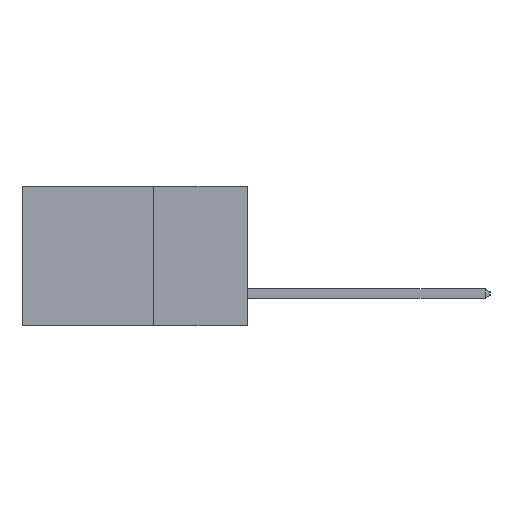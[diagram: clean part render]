
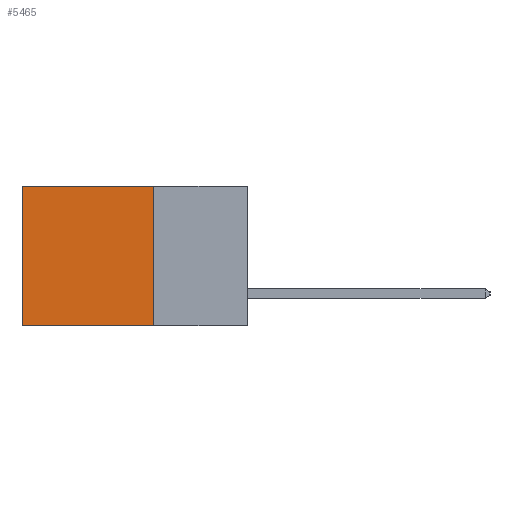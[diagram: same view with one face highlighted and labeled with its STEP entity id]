
A CAD part, left-side view. The second image highlights one B-rep face of the part: STEP entity #5465.
In plain terms, the highlighted planar face has unit normal (-1, 0, 0).
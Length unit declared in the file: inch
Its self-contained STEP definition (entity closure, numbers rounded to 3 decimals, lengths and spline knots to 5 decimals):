
#389 = ORIENTED_EDGE ( 'NONE', *, *, #894, .F. ) ;
#746 = LINE ( 'NONE', #4084, #8252 ) ;
#894 = EDGE_CURVE ( 'NONE', #5451, #9599, #11026, .T. ) ;
#908 = ORIENTED_EDGE ( 'NONE', *, *, #3267, .F. ) ;
#2327 = DIRECTION ( 'NONE',  ( 0., 0., -1. ) ) ;
#2341 = DIRECTION ( 'NONE',  ( 1., 0., 0. ) ) ;
#2351 = CARTESIAN_POINT ( 'NONE',  ( 0.2615, 0.25, -0.37 ) ) ;
#2366 = PLANE ( 'NONE',  #8957 ) ;
#2513 = CARTESIAN_POINT ( 'NONE',  ( 0.2615, 0.6, -0.37 ) ) ;
#2515 = ORIENTED_EDGE ( 'NONE', *, *, #6167, .T. ) ;
#2605 = CARTESIAN_POINT ( 'NONE',  ( 0.2615, 0.25, 0. ) ) ;
#3267 = EDGE_CURVE ( 'NONE', #9599, #12091, #746, .T. ) ;
#3925 = LINE ( 'NONE', #9229, #11230 ) ;
#4084 = CARTESIAN_POINT ( 'NONE',  ( 0.2615, 0.25, -0.37 ) ) ;
#4126 = CARTESIAN_POINT ( 'NONE',  ( 0.2615, 0.6, -0.37 ) ) ;
#4228 = DIRECTION ( 'NONE',  ( 0., 1., 0. ) ) ;
#5122 = DIRECTION ( 'NONE',  ( 0., 0., -1. ) ) ;
#5451 = VERTEX_POINT ( 'NONE', #2605 ) ;
#5465 = ADVANCED_FACE ( 'NONE', ( #9521 ), #2366, .F. ) ;
#6029 = CARTESIAN_POINT ( 'NONE',  ( 0.2615, 0.25, -0.37 ) ) ;
#6167 = EDGE_CURVE ( 'NONE', #5451, #9443, #3925, .T. ) ;
#6570 = CARTESIAN_POINT ( 'NONE',  ( 0.2615, 0.6, 0. ) ) ;
#8252 = VECTOR ( 'NONE', #4228, 39.37008 ) ;
#8491 = EDGE_LOOP ( 'NONE', ( #11199, #908, #389, #2515 ) ) ;
#8557 = VECTOR ( 'NONE', #10948, 39.37008 ) ;
#8957 = AXIS2_PLACEMENT_3D ( 'NONE', #2351, #2341, #2327 ) ;
#9148 = DIRECTION ( 'NONE',  ( 0., 1., 0. ) ) ;
#9225 = VECTOR ( 'NONE', #5122, 39.37008 ) ;
#9229 = CARTESIAN_POINT ( 'NONE',  ( 0.2615, 0.25, 0. ) ) ;
#9443 = VERTEX_POINT ( 'NONE', #6570 ) ;
#9521 = FACE_OUTER_BOUND ( 'NONE', #8491, .T. ) ;
#9599 = VERTEX_POINT ( 'NONE', #6029 ) ;
#10235 = CARTESIAN_POINT ( 'NONE',  ( 0.2615, 0.25, -0.37 ) ) ;
#10948 = DIRECTION ( 'NONE',  ( 0., 0., -1. ) ) ;
#11026 = LINE ( 'NONE', #10235, #8557 ) ;
#11199 = ORIENTED_EDGE ( 'NONE', *, *, #11892, .T. ) ;
#11230 = VECTOR ( 'NONE', #9148, 39.37008 ) ;
#11892 = EDGE_CURVE ( 'NONE', #9443, #12091, #11940, .T. ) ;
#11940 = LINE ( 'NONE', #4126, #9225 ) ;
#12091 = VERTEX_POINT ( 'NONE', #2513 ) ;
